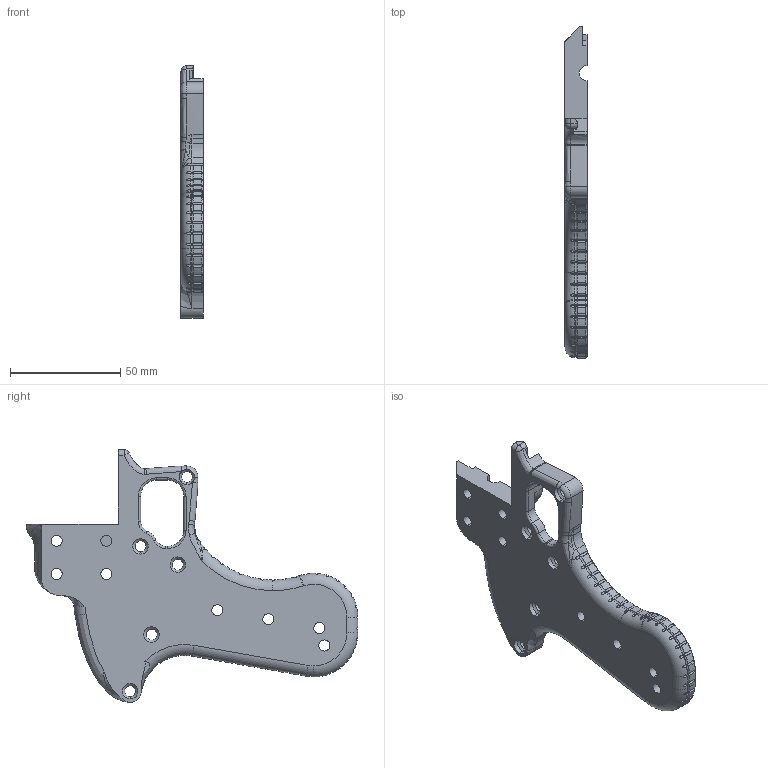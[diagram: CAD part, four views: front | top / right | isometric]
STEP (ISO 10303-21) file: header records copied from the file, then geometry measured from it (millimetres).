
FILE_DESCRIPTION (( 'STEP AP214' ), '1' );
FILE_NAME ('Side_Right.STEP', '2014-02-20T01:05:03', ( '' ), ( '' ), 'SwSTEP 2.0', 'SolidWorks 2013', '' );
FILE_SCHEMA (( 'AUTOMOTIVE_DESIGN' ));
Length unit declared in the file: millimetre
Products named in the file (1): Side_Right
Bounding box: 10 x 150.34 x 114.42 mm (x, y, z)
Volume: 49310.4 mm3; surface area: 23069.2 mm2
Topology: 1 solids, 1 shells, 492 faces, 1262 edges, 765 vertices
Faces by surface type: cylinder 285, torus 104, plane 61, bspline 29, cone 12, sphere 1
Entity records: 18313 total; most frequent: CARTESIAN_POINT 7105, ORIENTED_EDGE 2508, DIRECTION 2177, EDGE_CURVE 1254, AXIS2_PLACEMENT_3D 882, VERTEX_POINT 765, EDGE_LOOP 519, FACE_OUTER_BOUND 492
